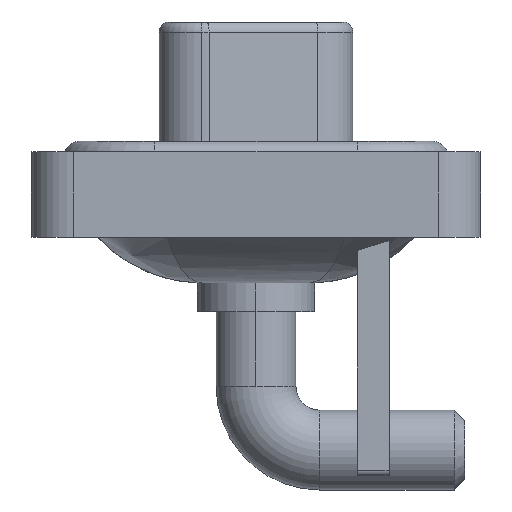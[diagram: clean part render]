
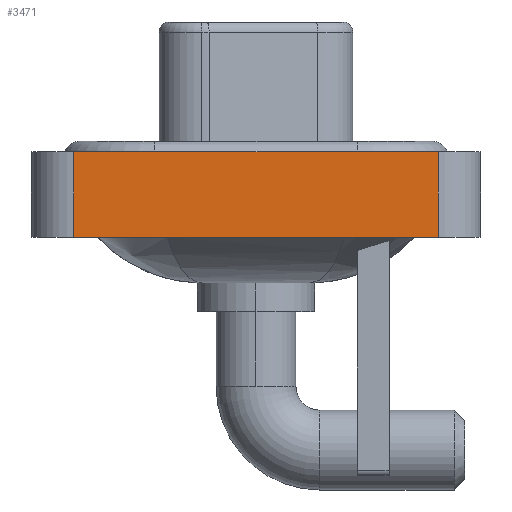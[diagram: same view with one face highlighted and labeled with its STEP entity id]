
A CAD part, left-side view. The second image highlights one B-rep face of the part: STEP entity #3471.
In plain terms, the highlighted planar face has unit normal (-1, 0, 0).
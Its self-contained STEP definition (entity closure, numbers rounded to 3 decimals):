
#890 = DIRECTION ( 'NONE',  ( 0., -1., 0. ) ) ;
#1741 = DIRECTION ( 'NONE',  ( 0., -1., 0. ) ) ;
#1816 = LINE ( 'NONE', #11312, #7907 ) ;
#2169 = EDGE_CURVE ( 'NONE', #6833, #8267, #1816, .T. ) ;
#3471 = ADVANCED_FACE ( 'NONE', ( #11735 ), #10252, .T. ) ;
#3887 = DIRECTION ( 'NONE',  ( 0., 0., 1. ) ) ;
#3981 = EDGE_CURVE ( 'NONE', #14052, #10508, #6219, .T. ) ;
#4124 = CARTESIAN_POINT ( 'NONE',  ( -7.3, 8.55, 0.4 ) ) ;
#4249 = AXIS2_PLACEMENT_3D ( 'NONE', #14280, #11571, #3887 ) ;
#5020 = EDGE_LOOP ( 'NONE', ( #16874, #17196, #5613, #11170 ) ) ;
#5613 = ORIENTED_EDGE ( 'NONE', *, *, #3981, .F. ) ;
#5904 = EDGE_CURVE ( 'NONE', #10508, #8267, #10719, .T. ) ;
#6219 = LINE ( 'NONE', #7779, #10952 ) ;
#6833 = VERTEX_POINT ( 'NONE', #11351 ) ;
#7608 = DIRECTION ( 'NONE',  ( 0., 0., 1. ) ) ;
#7635 = VECTOR ( 'NONE', #890, 1000. ) ;
#7779 = CARTESIAN_POINT ( 'NONE',  ( -7.3, 8.55, -3.6 ) ) ;
#7907 = VECTOR ( 'NONE', #8503, 1000. ) ;
#8267 = VERTEX_POINT ( 'NONE', #10371 ) ;
#8503 = DIRECTION ( 'NONE',  ( 0., 0., 1. ) ) ;
#8896 = CARTESIAN_POINT ( 'NONE',  ( -7.3, -8.55, -3.6 ) ) ;
#9964 = LINE ( 'NONE', #8896, #7635 ) ;
#10252 = PLANE ( 'NONE',  #4249 ) ;
#10371 = CARTESIAN_POINT ( 'NONE',  ( -7.3, -8.55, 0.4 ) ) ;
#10508 = VERTEX_POINT ( 'NONE', #4124 ) ;
#10559 = VECTOR ( 'NONE', #1741, 1000. ) ;
#10719 = LINE ( 'NONE', #12016, #10559 ) ;
#10952 = VECTOR ( 'NONE', #7608, 1000. ) ;
#11170 = ORIENTED_EDGE ( 'NONE', *, *, #12083, .T. ) ;
#11312 = CARTESIAN_POINT ( 'NONE',  ( -7.3, -8.55, -3.6 ) ) ;
#11351 = CARTESIAN_POINT ( 'NONE',  ( -7.3, -8.55, -3.6 ) ) ;
#11410 = CARTESIAN_POINT ( 'NONE',  ( -7.3, 8.55, -3.6 ) ) ;
#11571 = DIRECTION ( 'NONE',  ( -1., 0., 0. ) ) ;
#11735 = FACE_OUTER_BOUND ( 'NONE', #5020, .T. ) ;
#12016 = CARTESIAN_POINT ( 'NONE',  ( -7.3, -8.55, 0.4 ) ) ;
#12083 = EDGE_CURVE ( 'NONE', #14052, #6833, #9964, .T. ) ;
#14052 = VERTEX_POINT ( 'NONE', #11410 ) ;
#14280 = CARTESIAN_POINT ( 'NONE',  ( -7.3, -8.55, -3.6 ) ) ;
#16874 = ORIENTED_EDGE ( 'NONE', *, *, #2169, .T. ) ;
#17196 = ORIENTED_EDGE ( 'NONE', *, *, #5904, .F. ) ;
